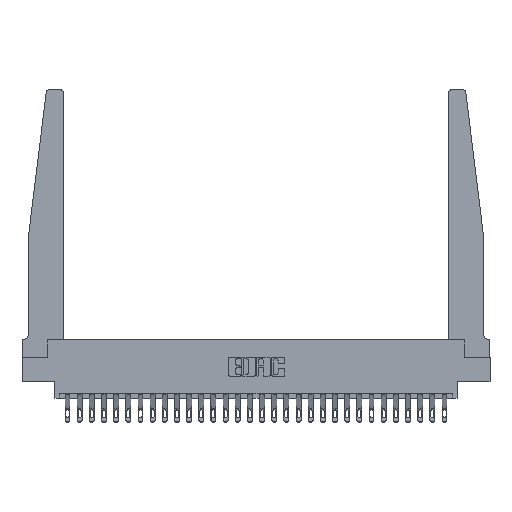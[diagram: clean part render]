
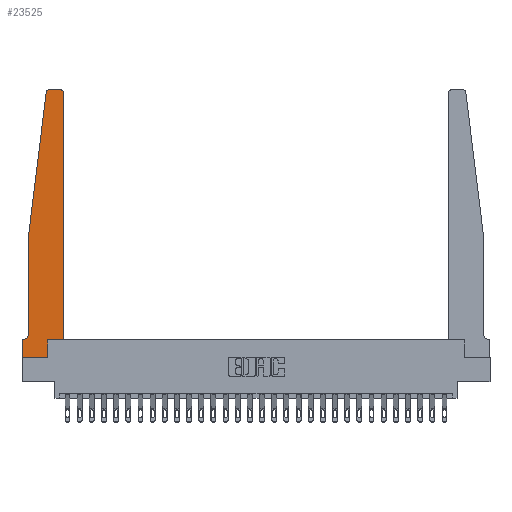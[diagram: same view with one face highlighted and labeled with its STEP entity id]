
A CAD part, top view. The second image highlights one B-rep face of the part: STEP entity #23525.
In plain terms, the highlighted planar face has unit normal (0, 0, 1).
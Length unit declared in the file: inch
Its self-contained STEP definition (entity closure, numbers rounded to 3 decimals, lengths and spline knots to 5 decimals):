
#49 = AXIS2_PLACEMENT_3D ( 'NONE', #24018, #26127, #13573 ) ;
#255 = VECTOR ( 'NONE', #13371, 39.37008 ) ;
#696 = EDGE_CURVE ( 'NONE', #25558, #7060, #7751, .T. ) ;
#1135 = DIRECTION ( 'NONE',  ( -1., 0., 0. ) ) ;
#1361 = DIRECTION ( 'NONE',  ( 1., 0., 0. ) ) ;
#1562 = CARTESIAN_POINT ( 'NONE',  ( 0.24675, 2.72367, 0.37 ) ) ;
#1635 = DIRECTION ( 'NONE',  ( -0.122, -0.992, 0. ) ) ;
#2064 = ORIENTED_EDGE ( 'NONE', *, *, #21017, .T. ) ;
#2608 = VERTEX_POINT ( 'NONE', #25074 ) ;
#3415 = ORIENTED_EDGE ( 'NONE', *, *, #19987, .T. ) ;
#3802 = VERTEX_POINT ( 'NONE', #18223 ) ;
#3842 = EDGE_CURVE ( 'NONE', #3802, #25558, #26061, .T. ) ;
#4000 = CARTESIAN_POINT ( 'NONE',  ( 0.065, 0.1875, 0.37 ) ) ;
#4101 = CARTESIAN_POINT ( 'NONE',  ( 0.065, 1.25, 0.37 ) ) ;
#4351 = CARTESIAN_POINT ( 'NONE',  ( 0., 0., 0.37 ) ) ;
#4758 = ORIENTED_EDGE ( 'NONE', *, *, #22067, .T. ) ;
#5875 = EDGE_CURVE ( 'NONE', #20428, #2608, #22812, .T. ) ;
#6248 = DIRECTION ( 'NONE',  ( 0., -1., 0. ) ) ;
#6250 = LINE ( 'NONE', #4000, #22468 ) ;
#6608 = VECTOR ( 'NONE', #22604, 39.37008 ) ;
#6746 = AXIS2_PLACEMENT_3D ( 'NONE', #20057, #7365, #22143 ) ;
#6818 = VERTEX_POINT ( 'NONE', #4351 ) ;
#7060 = VERTEX_POINT ( 'NONE', #17831 ) ;
#7109 = DIRECTION ( 'NONE',  ( 0., -1., 0. ) ) ;
#7149 = CIRCLE ( 'NONE', #16017, 0.03 ) ;
#7365 = DIRECTION ( 'NONE',  ( 0., 0., -1. ) ) ;
#7538 = CARTESIAN_POINT ( 'NONE',  ( 0.25, 2.75, 0.37 ) ) ;
#7751 = LINE ( 'NONE', #16592, #24571 ) ;
#8134 = ORIENTED_EDGE ( 'NONE', *, *, #5875, .T. ) ;
#8197 = VECTOR ( 'NONE', #7109, 39.37008 ) ;
#8728 = CARTESIAN_POINT ( 'NONE',  ( 0.395, 2.75, 0.37 ) ) ;
#9261 = CARTESIAN_POINT ( 'NONE',  ( 0., 0., 0.37 ) ) ;
#9289 = PLANE ( 'NONE',  #49 ) ;
#9508 = CARTESIAN_POINT ( 'NONE',  ( 0.395, 2.72, 0.37 ) ) ;
#9799 = CARTESIAN_POINT ( 'NONE',  ( 0.425, 0.18, 0.37 ) ) ;
#9984 = CARTESIAN_POINT ( 'NONE',  ( 0.425, 0.18, 0.37 ) ) ;
#10296 = VECTOR ( 'NONE', #17711, 39.37008 ) ;
#11145 = VERTEX_POINT ( 'NONE', #8728 ) ;
#11285 = EDGE_CURVE ( 'NONE', #23566, #15178, #17322, .T. ) ;
#11611 = DIRECTION ( 'NONE',  ( 1., 0., 0. ) ) ;
#13103 = FACE_OUTER_BOUND ( 'NONE', #13339, .T. ) ;
#13339 = EDGE_LOOP ( 'NONE', ( #2064, #19047, #19722, #3415, #20374, #21016, #4758, #22323, #22986, #23641, #8134, #19395 ) ) ;
#13371 = DIRECTION ( 'NONE',  ( 0., 1., 0. ) ) ;
#13573 = DIRECTION ( 'NONE',  ( 1., 0., 0. ) ) ;
#13965 = DIRECTION ( 'NONE',  ( 1., 0., 0. ) ) ;
#14182 = DIRECTION ( 'NONE',  ( 0., 0., 1. ) ) ;
#15178 = VERTEX_POINT ( 'NONE', #18752 ) ;
#15790 = CARTESIAN_POINT ( 'NONE',  ( 0.2605, 0., 0.37 ) ) ;
#15951 = LINE ( 'NONE', #23918, #10296 ) ;
#16017 = AXIS2_PLACEMENT_3D ( 'NONE', #9508, #24228, #11611 ) ;
#16130 = EDGE_CURVE ( 'NONE', #6818, #23566, #15951, .T. ) ;
#16470 = LINE ( 'NONE', #26423, #26942 ) ;
#16592 = CARTESIAN_POINT ( 'NONE',  ( 0.065, 1.25, 0.37 ) ) ;
#17322 = LINE ( 'NONE', #25943, #255 ) ;
#17711 = DIRECTION ( 'NONE',  ( 1., 0., 0. ) ) ;
#17831 = CARTESIAN_POINT ( 'NONE',  ( 0.065, 1.25, 0.37 ) ) ;
#17883 = LINE ( 'NONE', #7538, #22777 ) ;
#18223 = CARTESIAN_POINT ( 'NONE',  ( 0.27653, 2.75, 0.37 ) ) ;
#18752 = CARTESIAN_POINT ( 'NONE',  ( 0.2605, 0.18, 0.37 ) ) ;
#19047 = ORIENTED_EDGE ( 'NONE', *, *, #3842, .T. ) ;
#19395 = ORIENTED_EDGE ( 'NONE', *, *, #22827, .T. ) ;
#19722 = ORIENTED_EDGE ( 'NONE', *, *, #696, .T. ) ;
#19908 = LINE ( 'NONE', #4101, #25453 ) ;
#19987 = EDGE_CURVE ( 'NONE', #7060, #25183, #19908, .T. ) ;
#20057 = CARTESIAN_POINT ( 'NONE',  ( 0.015, 0.2375, 0.37 ) ) ;
#20374 = ORIENTED_EDGE ( 'NONE', *, *, #24233, .T. ) ;
#20428 = VERTEX_POINT ( 'NONE', #9799 ) ;
#21016 = ORIENTED_EDGE ( 'NONE', *, *, #26383, .T. ) ;
#21017 = EDGE_CURVE ( 'NONE', #11145, #3802, #17883, .T. ) ;
#21251 = AXIS2_PLACEMENT_3D ( 'NONE', #26729, #14182, #1361 ) ;
#22067 = EDGE_CURVE ( 'NONE', #22400, #6818, #25006, .T. ) ;
#22143 = DIRECTION ( 'NONE',  ( -1., 0., 0. ) ) ;
#22323 = ORIENTED_EDGE ( 'NONE', *, *, #16130, .T. ) ;
#22400 = VERTEX_POINT ( 'NONE', #22875 ) ;
#22468 = VECTOR ( 'NONE', #27198, 39.37008 ) ;
#22604 = DIRECTION ( 'NONE',  ( 0., 1., 0. ) ) ;
#22749 = CARTESIAN_POINT ( 'NONE',  ( 0.015, 0.1875, 0.37 ) ) ;
#22777 = VECTOR ( 'NONE', #1135, 39.37008 ) ;
#22812 = LINE ( 'NONE', #9984, #6608 ) ;
#22827 = EDGE_CURVE ( 'NONE', #2608, #11145, #7149, .T. ) ;
#22875 = CARTESIAN_POINT ( 'NONE',  ( 0., 0.1875, 0.37 ) ) ;
#22894 = EDGE_CURVE ( 'NONE', #15178, #20428, #16470, .T. ) ;
#22986 = ORIENTED_EDGE ( 'NONE', *, *, #11285, .T. ) ;
#23057 = VERTEX_POINT ( 'NONE', #22749 ) ;
#23525 = ADVANCED_FACE ( 'NONE', ( #13103 ), #9289, .T. ) ;
#23566 = VERTEX_POINT ( 'NONE', #15790 ) ;
#23641 = ORIENTED_EDGE ( 'NONE', *, *, #22894, .T. ) ;
#23911 = CIRCLE ( 'NONE', #6746, 0.05 ) ;
#23918 = CARTESIAN_POINT ( 'NONE',  ( 0., 0., 0.37 ) ) ;
#24018 = CARTESIAN_POINT ( 'NONE',  ( 0., 0.1875, 0.37 ) ) ;
#24228 = DIRECTION ( 'NONE',  ( 0., 0., 1. ) ) ;
#24233 = EDGE_CURVE ( 'NONE', #25183, #23057, #23911, .T. ) ;
#24571 = VECTOR ( 'NONE', #1635, 39.37008 ) ;
#25006 = LINE ( 'NONE', #9261, #8197 ) ;
#25074 = CARTESIAN_POINT ( 'NONE',  ( 0.425, 2.72, 0.37 ) ) ;
#25183 = VERTEX_POINT ( 'NONE', #25766 ) ;
#25453 = VECTOR ( 'NONE', #6248, 39.37008 ) ;
#25558 = VERTEX_POINT ( 'NONE', #1562 ) ;
#25766 = CARTESIAN_POINT ( 'NONE',  ( 0.065, 0.2375, 0.37 ) ) ;
#25943 = CARTESIAN_POINT ( 'NONE',  ( 0.2605, 0.18, 0.37 ) ) ;
#26061 = CIRCLE ( 'NONE', #21251, 0.03 ) ;
#26127 = DIRECTION ( 'NONE',  ( 0., 0., 1. ) ) ;
#26383 = EDGE_CURVE ( 'NONE', #23057, #22400, #6250, .T. ) ;
#26423 = CARTESIAN_POINT ( 'NONE',  ( 0.425, 0.18, 0.37 ) ) ;
#26729 = CARTESIAN_POINT ( 'NONE',  ( 0.27653, 2.72, 0.37 ) ) ;
#26942 = VECTOR ( 'NONE', #13965, 39.37008 ) ;
#27198 = DIRECTION ( 'NONE',  ( -1., 0., 0. ) ) ;
